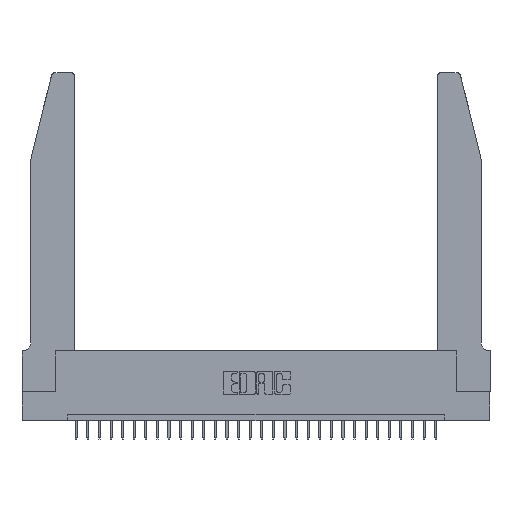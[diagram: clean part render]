
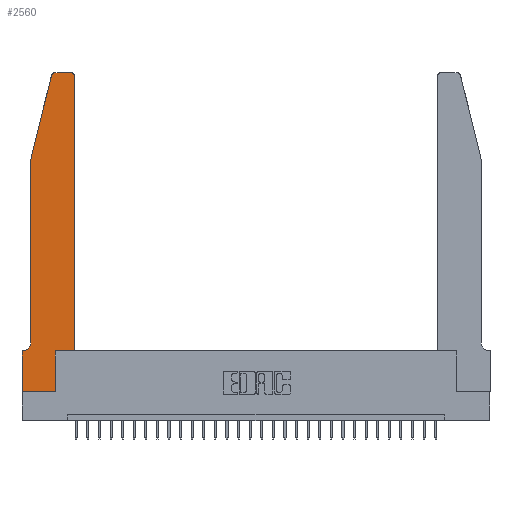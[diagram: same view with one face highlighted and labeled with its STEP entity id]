
A CAD part, top view. The second image highlights one B-rep face of the part: STEP entity #2560.
In plain terms, the highlighted planar face has unit normal (0, 0, 1).
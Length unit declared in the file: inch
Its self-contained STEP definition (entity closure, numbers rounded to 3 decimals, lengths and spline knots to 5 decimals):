
#90 = LINE ( 'NONE', #2367, #18013 ) ;
#173 = ORIENTED_EDGE ( 'NONE', *, *, #5141, .T. ) ;
#240 = LINE ( 'NONE', #18243, #21437 ) ;
#278 = DIRECTION ( 'NONE',  ( 1., 0., 0. ) ) ;
#408 = CARTESIAN_POINT ( 'NONE',  ( 0., 0., 0.37 ) ) ;
#449 = CIRCLE ( 'NONE', #22016, 0.03 ) ;
#787 = CARTESIAN_POINT ( 'NONE',  ( 0.2865, 0.35, 0.37 ) ) ;
#942 = PLANE ( 'NONE',  #23980 ) ;
#1087 = DIRECTION ( 'NONE',  ( 0., 0., -1. ) ) ;
#1177 = CARTESIAN_POINT ( 'NONE',  ( 0., 0.35, 0.37 ) ) ;
#1220 = DIRECTION ( 'NONE',  ( 1., 0., 0. ) ) ;
#1567 = DIRECTION ( 'NONE',  ( 0., -1., 0. ) ) ;
#1684 = LINE ( 'NONE', #787, #11897 ) ;
#1689 = VECTOR ( 'NONE', #10024, 39.37008 ) ;
#1758 = VERTEX_POINT ( 'NONE', #13556 ) ;
#2367 = CARTESIAN_POINT ( 'NONE',  ( 0.0755, 0.35, 0.37 ) ) ;
#2560 = ADVANCED_FACE ( 'NONE', ( #8665 ), #942, .T. ) ;
#2701 = VECTOR ( 'NONE', #22084, 39.37008 ) ;
#2726 = EDGE_CURVE ( 'NONE', #22995, #13266, #1684, .T. ) ;
#3108 = ORIENTED_EDGE ( 'NONE', *, *, #6805, .T. ) ;
#3609 = EDGE_CURVE ( 'NONE', #11170, #22995, #15947, .T. ) ;
#4729 = EDGE_CURVE ( 'NONE', #8712, #11170, #14363, .T. ) ;
#5141 = EDGE_CURVE ( 'NONE', #8181, #8712, #90, .T. ) ;
#5187 = DIRECTION ( 'NONE',  ( 0., 0., 1. ) ) ;
#5207 = CIRCLE ( 'NONE', #9073, 0.07 ) ;
#5847 = ORIENTED_EDGE ( 'NONE', *, *, #7714, .T. ) ;
#6207 = CARTESIAN_POINT ( 'NONE',  ( 0.4505, 0.35, 0.37 ) ) ;
#6601 = EDGE_LOOP ( 'NONE', ( #20541, #16789, #5847, #29217, #21814, #173, #14259, #19111, #30015, #19912, #3108, #25440 ) ) ;
#6805 = EDGE_CURVE ( 'NONE', #10996, #11273, #30287, .T. ) ;
#7629 = DIRECTION ( 'NONE',  ( 0., 1., 0. ) ) ;
#7671 = CARTESIAN_POINT ( 'NONE',  ( 0., 0., 0.37 ) ) ;
#7714 = EDGE_CURVE ( 'NONE', #27520, #20214, #27234, .T. ) ;
#8109 = VERTEX_POINT ( 'NONE', #11620 ) ;
#8181 = VERTEX_POINT ( 'NONE', #26041 ) ;
#8540 = EDGE_CURVE ( 'NONE', #8109, #27520, #22402, .T. ) ;
#8583 = EDGE_CURVE ( 'NONE', #1758, #8181, #5207, .T. ) ;
#8665 = FACE_OUTER_BOUND ( 'NONE', #6601, .T. ) ;
#8712 = VERTEX_POINT ( 'NONE', #1177 ) ;
#8998 = CARTESIAN_POINT ( 'NONE',  ( 0.4205, 2.75, 0.37 ) ) ;
#9073 = AXIS2_PLACEMENT_3D ( 'NONE', #19600, #1087, #17423 ) ;
#9131 = EDGE_CURVE ( 'NONE', #20214, #1758, #12509, .T. ) ;
#9171 = VERTEX_POINT ( 'NONE', #8998 ) ;
#10024 = DIRECTION ( 'NONE',  ( 1., 0., 0. ) ) ;
#10330 = CARTESIAN_POINT ( 'NONE',  ( 0., 0.35, 0.37 ) ) ;
#10532 = CARTESIAN_POINT ( 'NONE',  ( 0.4505, 2.72, 0.37 ) ) ;
#10996 = VERTEX_POINT ( 'NONE', #6207 ) ;
#11170 = VERTEX_POINT ( 'NONE', #7671 ) ;
#11185 = CARTESIAN_POINT ( 'NONE',  ( 0., 0., 0.37 ) ) ;
#11273 = VERTEX_POINT ( 'NONE', #10532 ) ;
#11620 = CARTESIAN_POINT ( 'NONE',  ( 0.284, 2.75, 0.37 ) ) ;
#11753 = DIRECTION ( 'NONE',  ( 0., 0., 1. ) ) ;
#11897 = VECTOR ( 'NONE', #7629, 39.37008 ) ;
#11941 = CARTESIAN_POINT ( 'NONE',  ( 0.4205, 2.72, 0.37 ) ) ;
#12131 = CARTESIAN_POINT ( 'NONE',  ( 0.284, 2.72, 0.37 ) ) ;
#12159 = DIRECTION ( 'NONE',  ( -1., 0., 0. ) ) ;
#12509 = LINE ( 'NONE', #12770, #17998 ) ;
#12770 = CARTESIAN_POINT ( 'NONE',  ( 0.0755, 2., 0.37 ) ) ;
#13266 = VERTEX_POINT ( 'NONE', #27788 ) ;
#13556 = CARTESIAN_POINT ( 'NONE',  ( 0.0755, 0.42, 0.37 ) ) ;
#13660 = CARTESIAN_POINT ( 'NONE',  ( 0.0755, 2., 0.37 ) ) ;
#14259 = ORIENTED_EDGE ( 'NONE', *, *, #4729, .T. ) ;
#14363 = LINE ( 'NONE', #11185, #22050 ) ;
#15682 = DIRECTION ( 'NONE',  ( -1., 0., 0. ) ) ;
#15793 = CARTESIAN_POINT ( 'NONE',  ( 0.2865, 0., 0.37 ) ) ;
#15894 = EDGE_CURVE ( 'NONE', #9171, #8109, #240, .T. ) ;
#15947 = LINE ( 'NONE', #408, #1689 ) ;
#15964 = CARTESIAN_POINT ( 'NONE',  ( 0.25487, 2.72718, 0.37 ) ) ;
#16789 = ORIENTED_EDGE ( 'NONE', *, *, #8540, .T. ) ;
#17423 = DIRECTION ( 'NONE',  ( -1., 0., 0. ) ) ;
#17441 = DIRECTION ( 'NONE',  ( 0., 1., 0. ) ) ;
#17769 = CARTESIAN_POINT ( 'NONE',  ( 0.4505, 0.35, 0.37 ) ) ;
#17998 = VECTOR ( 'NONE', #19829, 39.37008 ) ;
#18013 = VECTOR ( 'NONE', #12159, 39.37008 ) ;
#18243 = CARTESIAN_POINT ( 'NONE',  ( 0.2605, 2.75, 0.37 ) ) ;
#19111 = ORIENTED_EDGE ( 'NONE', *, *, #3609, .T. ) ;
#19366 = EDGE_CURVE ( 'NONE', #13266, #10996, #28925, .T. ) ;
#19512 = CARTESIAN_POINT ( 'NONE',  ( 0.4505, 0.35, 0.37 ) ) ;
#19600 = CARTESIAN_POINT ( 'NONE',  ( 0.0055, 0.42, 0.37 ) ) ;
#19829 = DIRECTION ( 'NONE',  ( 0., -1., 0. ) ) ;
#19912 = ORIENTED_EDGE ( 'NONE', *, *, #19366, .T. ) ;
#20214 = VERTEX_POINT ( 'NONE', #13660 ) ;
#20541 = ORIENTED_EDGE ( 'NONE', *, *, #15894, .T. ) ;
#20613 = AXIS2_PLACEMENT_3D ( 'NONE', #12131, #5187, #278 ) ;
#21437 = VECTOR ( 'NONE', #15682, 39.37008 ) ;
#21814 = ORIENTED_EDGE ( 'NONE', *, *, #8583, .T. ) ;
#22016 = AXIS2_PLACEMENT_3D ( 'NONE', #11941, #11753, #23610 ) ;
#22050 = VECTOR ( 'NONE', #1567, 39.37008 ) ;
#22084 = DIRECTION ( 'NONE',  ( -0.239, -0.971, 0. ) ) ;
#22402 = CIRCLE ( 'NONE', #20613, 0.03 ) ;
#22995 = VERTEX_POINT ( 'NONE', #15793 ) ;
#23456 = VECTOR ( 'NONE', #1220, 39.37008 ) ;
#23610 = DIRECTION ( 'NONE',  ( 1., 0., 0. ) ) ;
#23980 = AXIS2_PLACEMENT_3D ( 'NONE', #10330, #28935, #28841 ) ;
#25440 = ORIENTED_EDGE ( 'NONE', *, *, #27751, .T. ) ;
#26041 = CARTESIAN_POINT ( 'NONE',  ( 0.0055, 0.35, 0.37 ) ) ;
#26670 = VECTOR ( 'NONE', #17441, 39.37008 ) ;
#27234 = LINE ( 'NONE', #29958, #2701 ) ;
#27520 = VERTEX_POINT ( 'NONE', #15964 ) ;
#27751 = EDGE_CURVE ( 'NONE', #11273, #9171, #449, .T. ) ;
#27788 = CARTESIAN_POINT ( 'NONE',  ( 0.2865, 0.35, 0.37 ) ) ;
#28841 = DIRECTION ( 'NONE',  ( 1., 0., 0. ) ) ;
#28925 = LINE ( 'NONE', #17769, #23456 ) ;
#28935 = DIRECTION ( 'NONE',  ( 0., 0., 1. ) ) ;
#29217 = ORIENTED_EDGE ( 'NONE', *, *, #9131, .T. ) ;
#29958 = CARTESIAN_POINT ( 'NONE',  ( 0.0755, 2., 0.37 ) ) ;
#30015 = ORIENTED_EDGE ( 'NONE', *, *, #2726, .T. ) ;
#30287 = LINE ( 'NONE', #19512, #26670 ) ;
